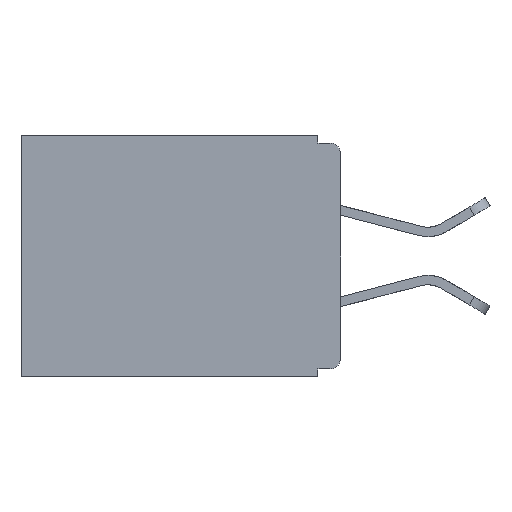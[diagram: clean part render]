
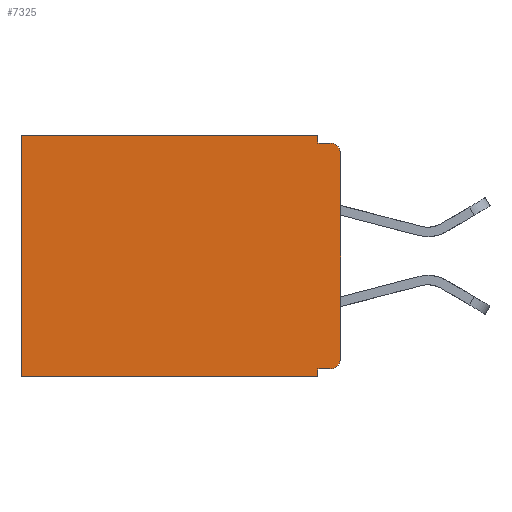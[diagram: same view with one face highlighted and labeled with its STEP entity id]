
A CAD part, left-side view. The second image highlights one B-rep face of the part: STEP entity #7325.
In plain terms, the highlighted planar face has unit normal (-1, 0, 0).
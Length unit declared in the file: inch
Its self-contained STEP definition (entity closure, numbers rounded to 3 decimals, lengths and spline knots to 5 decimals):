
#939 = CARTESIAN_POINT ( 'NONE',  ( 0.3, 0.031, 0. ) ) ;
#987 = EDGE_CURVE ( 'NONE', #19303, #9738, #9098, .T. ) ;
#1872 = VERTEX_POINT ( 'NONE', #2406 ) ;
#2056 = PLANE ( 'NONE',  #19216 ) ;
#2324 = ORIENTED_EDGE ( 'NONE', *, *, #12807, .F. ) ;
#2406 = CARTESIAN_POINT ( 'NONE',  ( 0.3, 0.031, -0.32 ) ) ;
#2668 = CARTESIAN_POINT ( 'NONE',  ( 0.3, 0.015, -0.01 ) ) ;
#3332 = CARTESIAN_POINT ( 'NONE',  ( 0.3, 0.015, -0.305 ) ) ;
#3720 = EDGE_CURVE ( 'NONE', #12666, #1872, #4067, .T. ) ;
#4016 = EDGE_CURVE ( 'NONE', #24626, #4783, #7150, .T. ) ;
#4067 = LINE ( 'NONE', #13658, #24080 ) ;
#4686 = DIRECTION ( 'NONE',  ( 0., -1., 0. ) ) ;
#4783 = VERTEX_POINT ( 'NONE', #23365 ) ;
#4877 = LINE ( 'NONE', #15099, #14699 ) ;
#5998 = ORIENTED_EDGE ( 'NONE', *, *, #20426, .T. ) ;
#6039 = CARTESIAN_POINT ( 'NONE',  ( 0.3, 0., -0.33 ) ) ;
#6162 = EDGE_CURVE ( 'NONE', #12666, #21966, #24243, .T. ) ;
#6192 = VECTOR ( 'NONE', #4686, 39.37008 ) ;
#6509 = DIRECTION ( 'NONE',  ( -1., 0., 0. ) ) ;
#6753 = CARTESIAN_POINT ( 'NONE',  ( 0.3, 0.031, -0.33 ) ) ;
#6794 = EDGE_LOOP ( 'NONE', ( #8481, #21199, #2324, #22385, #15191, #5998, #15534, #11576, #21829, #19160 ) ) ;
#6987 = DIRECTION ( 'NONE',  ( 0., 1., 0. ) ) ;
#7064 = DIRECTION ( 'NONE',  ( 0., 1., 0. ) ) ;
#7095 = CARTESIAN_POINT ( 'NONE',  ( 0.3, 0., -0.33 ) ) ;
#7150 = LINE ( 'NONE', #20267, #16884 ) ;
#7325 = ADVANCED_FACE ( 'NONE', ( #22806 ), #2056, .F. ) ;
#8481 = ORIENTED_EDGE ( 'NONE', *, *, #24667, .F. ) ;
#8501 = VECTOR ( 'NONE', #6987, 39.37008 ) ;
#8659 = CARTESIAN_POINT ( 'NONE',  ( 0.3, 0., -0.01 ) ) ;
#9098 = LINE ( 'NONE', #6039, #8501 ) ;
#9619 = AXIS2_PLACEMENT_3D ( 'NONE', #18173, #6509, #20105 ) ;
#9738 = VERTEX_POINT ( 'NONE', #15046 ) ;
#11268 = LINE ( 'NONE', #22325, #20342 ) ;
#11565 = DIRECTION ( 'NONE',  ( 0., 1., 0. ) ) ;
#11576 = ORIENTED_EDGE ( 'NONE', *, *, #11613, .F. ) ;
#11613 = EDGE_CURVE ( 'NONE', #1872, #19303, #11799, .T. ) ;
#11799 = LINE ( 'NONE', #6753, #16935 ) ;
#11882 = CIRCLE ( 'NONE', #9619, 0.015 ) ;
#12666 = VERTEX_POINT ( 'NONE', #18022 ) ;
#12807 = EDGE_CURVE ( 'NONE', #23054, #15497, #21075, .T. ) ;
#13127 = DIRECTION ( 'NONE',  ( 1., 0., 0. ) ) ;
#13186 = DIRECTION ( 'NONE',  ( 0., 0., -1. ) ) ;
#13520 = CARTESIAN_POINT ( 'NONE',  ( 0.3, 0.031, -0.01 ) ) ;
#13658 = CARTESIAN_POINT ( 'NONE',  ( 0.3, 0., -0.32 ) ) ;
#14699 = VECTOR ( 'NONE', #17037, 39.37008 ) ;
#15046 = CARTESIAN_POINT ( 'NONE',  ( 0.3, 0.437, -0.33 ) ) ;
#15099 = CARTESIAN_POINT ( 'NONE',  ( 0.3, 0.437, -0.33 ) ) ;
#15191 = ORIENTED_EDGE ( 'NONE', *, *, #4016, .T. ) ;
#15497 = VERTEX_POINT ( 'NONE', #2668 ) ;
#15534 = ORIENTED_EDGE ( 'NONE', *, *, #987, .F. ) ;
#15667 = LINE ( 'NONE', #7095, #20768 ) ;
#16802 = VERTEX_POINT ( 'NONE', #19679 ) ;
#16884 = VECTOR ( 'NONE', #11565, 39.37008 ) ;
#16935 = VECTOR ( 'NONE', #22215, 39.37008 ) ;
#17037 = DIRECTION ( 'NONE',  ( 0., 0., -1. ) ) ;
#17050 = EDGE_CURVE ( 'NONE', #24626, #23054, #11268, .T. ) ;
#18022 = CARTESIAN_POINT ( 'NONE',  ( 0.3, 0.015, -0.32 ) ) ;
#18173 = CARTESIAN_POINT ( 'NONE',  ( 0.3, 0.015, -0.025 ) ) ;
#18576 = DIRECTION ( 'NONE',  ( 0., 0., -1. ) ) ;
#18727 = DIRECTION ( 'NONE',  ( 0., 0., -1. ) ) ;
#19160 = ORIENTED_EDGE ( 'NONE', *, *, #6162, .T. ) ;
#19216 = AXIS2_PLACEMENT_3D ( 'NONE', #24593, #13127, #13186 ) ;
#19303 = VERTEX_POINT ( 'NONE', #22921 ) ;
#19679 = CARTESIAN_POINT ( 'NONE',  ( 0.3, 0., -0.025 ) ) ;
#19799 = DIRECTION ( 'NONE',  ( 0., 0., -1. ) ) ;
#20105 = DIRECTION ( 'NONE',  ( 0., 0., -1. ) ) ;
#20267 = CARTESIAN_POINT ( 'NONE',  ( 0.3, 0., 0. ) ) ;
#20342 = VECTOR ( 'NONE', #18576, 39.37008 ) ;
#20426 = EDGE_CURVE ( 'NONE', #4783, #9738, #4877, .T. ) ;
#20768 = VECTOR ( 'NONE', #18727, 39.37008 ) ;
#21075 = LINE ( 'NONE', #8659, #6192 ) ;
#21124 = AXIS2_PLACEMENT_3D ( 'NONE', #3332, #22318, #19799 ) ;
#21199 = ORIENTED_EDGE ( 'NONE', *, *, #22090, .T. ) ;
#21613 = CARTESIAN_POINT ( 'NONE',  ( 0.3, 0., -0.305 ) ) ;
#21829 = ORIENTED_EDGE ( 'NONE', *, *, #3720, .F. ) ;
#21966 = VERTEX_POINT ( 'NONE', #21613 ) ;
#22090 = EDGE_CURVE ( 'NONE', #16802, #15497, #11882, .T. ) ;
#22215 = DIRECTION ( 'NONE',  ( 0., 0., -1. ) ) ;
#22318 = DIRECTION ( 'NONE',  ( -1., 0., 0. ) ) ;
#22325 = CARTESIAN_POINT ( 'NONE',  ( 0.3, 0.031, 0. ) ) ;
#22385 = ORIENTED_EDGE ( 'NONE', *, *, #17050, .F. ) ;
#22806 = FACE_OUTER_BOUND ( 'NONE', #6794, .T. ) ;
#22921 = CARTESIAN_POINT ( 'NONE',  ( 0.3, 0.031, -0.33 ) ) ;
#23054 = VERTEX_POINT ( 'NONE', #13520 ) ;
#23365 = CARTESIAN_POINT ( 'NONE',  ( 0.3, 0.437, 0. ) ) ;
#24080 = VECTOR ( 'NONE', #7064, 39.37008 ) ;
#24243 = CIRCLE ( 'NONE', #21124, 0.015 ) ;
#24593 = CARTESIAN_POINT ( 'NONE',  ( 0.3, 0., -0.33 ) ) ;
#24626 = VERTEX_POINT ( 'NONE', #939 ) ;
#24667 = EDGE_CURVE ( 'NONE', #16802, #21966, #15667, .T. ) ;
